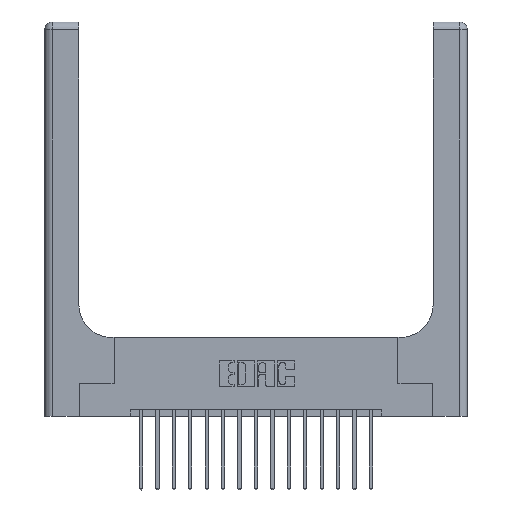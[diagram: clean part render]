
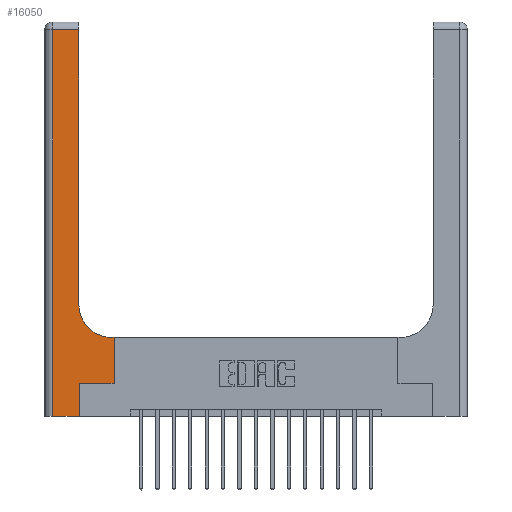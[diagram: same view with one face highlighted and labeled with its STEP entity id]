
A CAD part, top view. The second image highlights one B-rep face of the part: STEP entity #16050.
In plain terms, the highlighted planar face has unit normal (0, 0, 1).
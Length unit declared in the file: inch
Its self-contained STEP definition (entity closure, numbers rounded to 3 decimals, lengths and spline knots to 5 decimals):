
#99 = AXIS2_PLACEMENT_3D ( 'NONE', #12780, #11392, #11215 ) ;
#180 = VECTOR ( 'NONE', #16175, 39.37008 ) ;
#351 = CARTESIAN_POINT ( 'NONE',  ( 0.06, 2.94, 0.37 ) ) ;
#585 = EDGE_CURVE ( 'NONE', #11159, #7470, #5875, .T. ) ;
#795 = CARTESIAN_POINT ( 'NONE',  ( 0.528, 0.6, 0.37 ) ) ;
#1198 = AXIS2_PLACEMENT_3D ( 'NONE', #17453, #12145, #14637 ) ;
#1286 = CARTESIAN_POINT ( 'NONE',  ( 0.265, 0.25, 0.37 ) ) ;
#1334 = DIRECTION ( 'NONE',  ( 0., -1., 0. ) ) ;
#1368 = PLANE ( 'NONE',  #99 ) ;
#1699 = CIRCLE ( 'NONE', #1198, 0.25 ) ;
#2046 = LINE ( 'NONE', #6196, #9021 ) ;
#2199 = VERTEX_POINT ( 'NONE', #4476 ) ;
#2454 = LINE ( 'NONE', #17056, #8044 ) ;
#2968 = DIRECTION ( 'NONE',  ( 0., 1., 0. ) ) ;
#3522 = VERTEX_POINT ( 'NONE', #795 ) ;
#3884 = CARTESIAN_POINT ( 'NONE',  ( 0., 2.94, 0.37 ) ) ;
#4349 = ORIENTED_EDGE ( 'NONE', *, *, #585, .T. ) ;
#4476 = CARTESIAN_POINT ( 'NONE',  ( 0.26, 2.94, 0.37 ) ) ;
#4767 = EDGE_CURVE ( 'NONE', #8920, #5571, #16140, .T. ) ;
#5110 = CARTESIAN_POINT ( 'NONE',  ( 0.26, 0.85, 0.37 ) ) ;
#5525 = EDGE_CURVE ( 'NONE', #3522, #17114, #9973, .T. ) ;
#5571 = VERTEX_POINT ( 'NONE', #1286 ) ;
#5643 = DIRECTION ( 'NONE',  ( 1., 0., 0. ) ) ;
#5875 = LINE ( 'NONE', #8465, #7441 ) ;
#6165 = VECTOR ( 'NONE', #16788, 39.37008 ) ;
#6196 = CARTESIAN_POINT ( 'NONE',  ( 0.26, 3., 0.37 ) ) ;
#6402 = EDGE_CURVE ( 'NONE', #2199, #11159, #9275, .T. ) ;
#6647 = EDGE_CURVE ( 'NONE', #7470, #8920, #2454, .T. ) ;
#7231 = CARTESIAN_POINT ( 'NONE',  ( 0.265, 0., 0.37 ) ) ;
#7366 = EDGE_CURVE ( 'NONE', #13077, #3522, #15285, .T. ) ;
#7380 = CARTESIAN_POINT ( 'NONE',  ( 0.528, 0.25, 0.37 ) ) ;
#7441 = VECTOR ( 'NONE', #1334, 39.37008 ) ;
#7470 = VERTEX_POINT ( 'NONE', #17653 ) ;
#7576 = DIRECTION ( 'NONE',  ( 0., 1., 0. ) ) ;
#7696 = VERTEX_POINT ( 'NONE', #5110 ) ;
#7744 = FACE_OUTER_BOUND ( 'NONE', #13469, .T. ) ;
#8044 = VECTOR ( 'NONE', #18510, 39.37008 ) ;
#8465 = CARTESIAN_POINT ( 'NONE',  ( 0.06, 3., 0.37 ) ) ;
#8503 = ORIENTED_EDGE ( 'NONE', *, *, #12133, .T. ) ;
#8920 = VERTEX_POINT ( 'NONE', #15368 ) ;
#9021 = VECTOR ( 'NONE', #7576, 39.37008 ) ;
#9275 = LINE ( 'NONE', #3884, #15831 ) ;
#9973 = LINE ( 'NONE', #17720, #6165 ) ;
#11159 = VERTEX_POINT ( 'NONE', #351 ) ;
#11185 = CARTESIAN_POINT ( 'NONE',  ( 0.265, 0.25, 0.37 ) ) ;
#11215 = DIRECTION ( 'NONE',  ( -1., 0., 0. ) ) ;
#11392 = DIRECTION ( 'NONE',  ( 0., 0., -1. ) ) ;
#11781 = CARTESIAN_POINT ( 'NONE',  ( 0.528, 0.25, 0.37 ) ) ;
#12133 = EDGE_CURVE ( 'NONE', #7696, #2199, #2046, .T. ) ;
#12145 = DIRECTION ( 'NONE',  ( 0., 0., -1. ) ) ;
#12409 = ORIENTED_EDGE ( 'NONE', *, *, #7366, .T. ) ;
#12653 = ORIENTED_EDGE ( 'NONE', *, *, #16302, .T. ) ;
#12780 = CARTESIAN_POINT ( 'NONE',  ( 0., 3., 0.37 ) ) ;
#13077 = VERTEX_POINT ( 'NONE', #11781 ) ;
#13135 = ORIENTED_EDGE ( 'NONE', *, *, #4767, .T. ) ;
#13469 = EDGE_LOOP ( 'NONE', ( #8503, #17015, #4349, #14453, #13135, #18148, #12409, #15843, #12653 ) ) ;
#14089 = VECTOR ( 'NONE', #2968, 39.37008 ) ;
#14147 = DIRECTION ( 'NONE',  ( -1., 0., 0. ) ) ;
#14443 = VECTOR ( 'NONE', #5643, 39.37008 ) ;
#14453 = ORIENTED_EDGE ( 'NONE', *, *, #6647, .T. ) ;
#14637 = DIRECTION ( 'NONE',  ( 1., 0., 0. ) ) ;
#15285 = LINE ( 'NONE', #7380, #180 ) ;
#15368 = CARTESIAN_POINT ( 'NONE',  ( 0.265, 0., 0.37 ) ) ;
#15831 = VECTOR ( 'NONE', #14147, 39.37008 ) ;
#15843 = ORIENTED_EDGE ( 'NONE', *, *, #5525, .T. ) ;
#16050 = ADVANCED_FACE ( 'NONE', ( #7744 ), #1368, .F. ) ;
#16140 = LINE ( 'NONE', #7231, #14089 ) ;
#16175 = DIRECTION ( 'NONE',  ( 0., 1., 0. ) ) ;
#16302 = EDGE_CURVE ( 'NONE', #17114, #7696, #1699, .T. ) ;
#16788 = DIRECTION ( 'NONE',  ( -1., 0., 0. ) ) ;
#17015 = ORIENTED_EDGE ( 'NONE', *, *, #6402, .T. ) ;
#17056 = CARTESIAN_POINT ( 'NONE',  ( 0., 0., 0.37 ) ) ;
#17114 = VERTEX_POINT ( 'NONE', #17359 ) ;
#17359 = CARTESIAN_POINT ( 'NONE',  ( 0.51, 0.6, 0.37 ) ) ;
#17453 = CARTESIAN_POINT ( 'NONE',  ( 0.51, 0.85, 0.37 ) ) ;
#17653 = CARTESIAN_POINT ( 'NONE',  ( 0.06, 0., 0.37 ) ) ;
#17720 = CARTESIAN_POINT ( 'NONE',  ( 0.26, 0.6, 0.37 ) ) ;
#18148 = ORIENTED_EDGE ( 'NONE', *, *, #18563, .T. ) ;
#18276 = LINE ( 'NONE', #11185, #14443 ) ;
#18510 = DIRECTION ( 'NONE',  ( 1., 0., 0. ) ) ;
#18563 = EDGE_CURVE ( 'NONE', #5571, #13077, #18276, .T. ) ;
